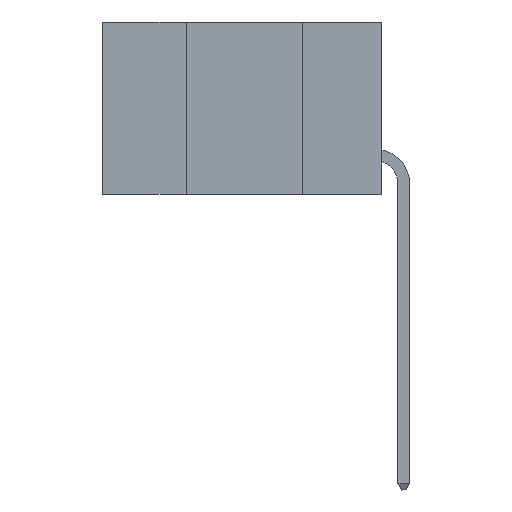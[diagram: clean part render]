
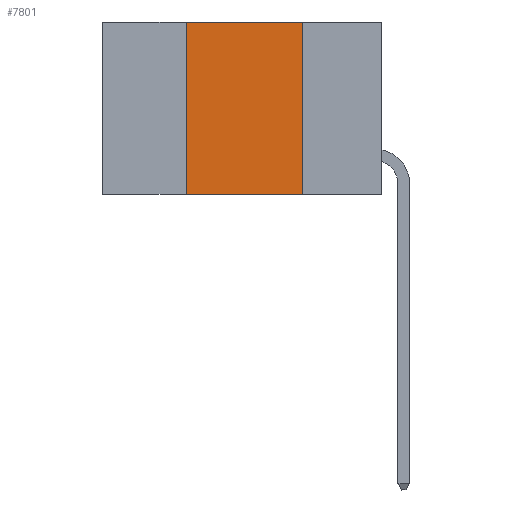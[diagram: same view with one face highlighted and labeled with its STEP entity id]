
A CAD part, left-side view. The second image highlights one B-rep face of the part: STEP entity #7801.
In plain terms, the highlighted planar face has unit normal (-1, 0, 0).
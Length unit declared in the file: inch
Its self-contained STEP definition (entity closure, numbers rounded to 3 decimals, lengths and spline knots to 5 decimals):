
#113 = EDGE_CURVE ( 'NONE', #746, #8368, #6670, .T. ) ;
#231 = VERTEX_POINT ( 'NONE', #4990 ) ;
#293 = DIRECTION ( 'NONE',  ( 0., 0., -1. ) ) ;
#425 = LINE ( 'NONE', #4764, #1745 ) ;
#477 = CARTESIAN_POINT ( 'NONE',  ( 0., 0.42, 0. ) ) ;
#738 = DIRECTION ( 'NONE',  ( 0., 0., -1. ) ) ;
#746 = VERTEX_POINT ( 'NONE', #8226 ) ;
#1593 = CARTESIAN_POINT ( 'NONE',  ( 0., 0.42, 0. ) ) ;
#1745 = VECTOR ( 'NONE', #3127, 39.37008 ) ;
#2911 = ORIENTED_EDGE ( 'NONE', *, *, #113, .F. ) ;
#3127 = DIRECTION ( 'NONE',  ( 0., -1., 0. ) ) ;
#3438 = CARTESIAN_POINT ( 'NONE',  ( 0., 0.17, 0. ) ) ;
#3522 = EDGE_CURVE ( 'NONE', #231, #8358, #9851, .T. ) ;
#3615 = AXIS2_PLACEMENT_3D ( 'NONE', #8649, #8904, #738 ) ;
#3784 = VECTOR ( 'NONE', #5170, 39.37008 ) ;
#4108 = DIRECTION ( 'NONE',  ( 0., 0., 1. ) ) ;
#4604 = EDGE_CURVE ( 'NONE', #8368, #231, #10619, .T. ) ;
#4684 = ORIENTED_EDGE ( 'NONE', *, *, #7458, .T. ) ;
#4764 = CARTESIAN_POINT ( 'NONE',  ( 0., 0.6, -0.37 ) ) ;
#4990 = CARTESIAN_POINT ( 'NONE',  ( 0., 0.17, 0. ) ) ;
#5170 = DIRECTION ( 'NONE',  ( 0., -1., 0. ) ) ;
#5370 = CARTESIAN_POINT ( 'NONE',  ( 0., 0.17, -0.37 ) ) ;
#6670 = LINE ( 'NONE', #1593, #10728 ) ;
#6729 = CARTESIAN_POINT ( 'NONE',  ( 0., 0.6, 0. ) ) ;
#6879 = EDGE_LOOP ( 'NONE', ( #9277, #8301, #2911, #4684 ) ) ;
#6968 = PLANE ( 'NONE',  #3615 ) ;
#7458 = EDGE_CURVE ( 'NONE', #746, #8358, #425, .T. ) ;
#7628 = VECTOR ( 'NONE', #293, 39.37008 ) ;
#7801 = ADVANCED_FACE ( 'NONE', ( #10296 ), #6968, .F. ) ;
#8226 = CARTESIAN_POINT ( 'NONE',  ( 0., 0.42, -0.37 ) ) ;
#8301 = ORIENTED_EDGE ( 'NONE', *, *, #4604, .F. ) ;
#8358 = VERTEX_POINT ( 'NONE', #5370 ) ;
#8368 = VERTEX_POINT ( 'NONE', #477 ) ;
#8649 = CARTESIAN_POINT ( 'NONE',  ( 0., 0.6, 0. ) ) ;
#8904 = DIRECTION ( 'NONE',  ( 1., 0., 0. ) ) ;
#9277 = ORIENTED_EDGE ( 'NONE', *, *, #3522, .F. ) ;
#9851 = LINE ( 'NONE', #3438, #7628 ) ;
#10296 = FACE_OUTER_BOUND ( 'NONE', #6879, .T. ) ;
#10619 = LINE ( 'NONE', #6729, #3784 ) ;
#10728 = VECTOR ( 'NONE', #4108, 39.37008 ) ;
